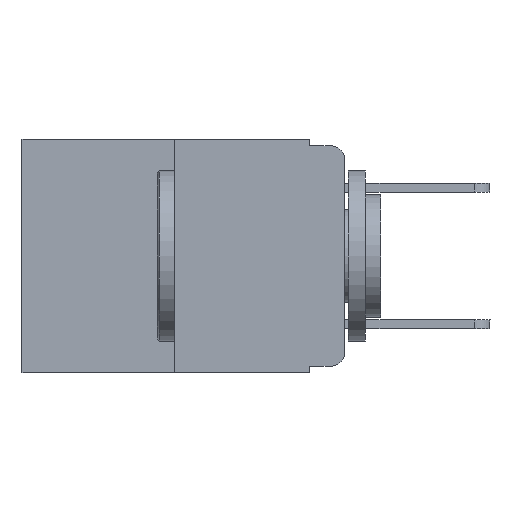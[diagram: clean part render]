
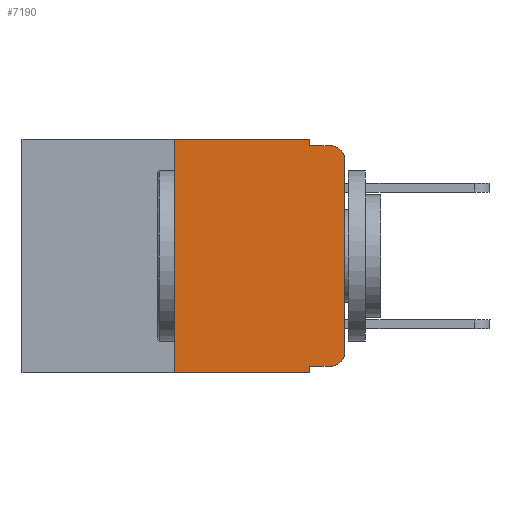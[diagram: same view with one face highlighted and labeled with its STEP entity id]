
A CAD part, left-side view. The second image highlights one B-rep face of the part: STEP entity #7190.
In plain terms, the highlighted planar face has unit normal (-1, 0, 0).
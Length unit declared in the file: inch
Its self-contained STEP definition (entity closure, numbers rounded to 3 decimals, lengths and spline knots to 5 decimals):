
#193 = CARTESIAN_POINT ( 'NONE',  ( 0., 0.02, -0.313 ) ) ;
#460 = VERTEX_POINT ( 'NONE', #11125 ) ;
#508 = VERTEX_POINT ( 'NONE', #9823 ) ;
#718 = DIRECTION ( 'NONE',  ( 0., -1., 0. ) ) ;
#870 = EDGE_CURVE ( 'NONE', #508, #15405, #17935, .T. ) ;
#947 = LINE ( 'NONE', #13880, #9600 ) ;
#1258 = EDGE_CURVE ( 'NONE', #11883, #17985, #17690, .T. ) ;
#1527 = LINE ( 'NONE', #17153, #15205 ) ;
#1578 = CARTESIAN_POINT ( 'NONE',  ( 0., 0.051, -0.01 ) ) ;
#1910 = ORIENTED_EDGE ( 'NONE', *, *, #1258, .T. ) ;
#2192 = VERTEX_POINT ( 'NONE', #6636 ) ;
#2486 = PLANE ( 'NONE',  #17309 ) ;
#2539 = CARTESIAN_POINT ( 'NONE',  ( 0., 0., -0.03 ) ) ;
#2745 = DIRECTION ( 'NONE',  ( 0., 0., -1. ) ) ;
#3162 = AXIS2_PLACEMENT_3D ( 'NONE', #193, #15656, #2745 ) ;
#3366 = ORIENTED_EDGE ( 'NONE', *, *, #870, .F. ) ;
#3822 = CARTESIAN_POINT ( 'NONE',  ( 0., 0.051, 0. ) ) ;
#4148 = ORIENTED_EDGE ( 'NONE', *, *, #4286, .F. ) ;
#4286 = EDGE_CURVE ( 'NONE', #15405, #4736, #947, .T. ) ;
#4331 = VECTOR ( 'NONE', #15826, 39.37008 ) ;
#4390 = EDGE_LOOP ( 'NONE', ( #16027, #1910, #17393, #4148, #3366, #5200, #5851, #8455, #18119, #8531 ) ) ;
#4405 = CARTESIAN_POINT ( 'NONE',  ( 0., 0., 0. ) ) ;
#4572 = CARTESIAN_POINT ( 'NONE',  ( 0., 0.051, -0.343 ) ) ;
#4736 = VERTEX_POINT ( 'NONE', #1578 ) ;
#4780 = EDGE_CURVE ( 'NONE', #4736, #17985, #13014, .T. ) ;
#4864 = DIRECTION ( 'NONE',  ( 0., -1., 0. ) ) ;
#4869 = AXIS2_PLACEMENT_3D ( 'NONE', #10899, #5118, #13799 ) ;
#5096 = VERTEX_POINT ( 'NONE', #18130 ) ;
#5118 = DIRECTION ( 'NONE',  ( -1., 0., 0. ) ) ;
#5120 = VECTOR ( 'NONE', #718, 39.37008 ) ;
#5200 = ORIENTED_EDGE ( 'NONE', *, *, #10684, .F. ) ;
#5493 = FACE_OUTER_BOUND ( 'NONE', #4390, .T. ) ;
#5517 = LINE ( 'NONE', #3822, #9323 ) ;
#5851 = ORIENTED_EDGE ( 'NONE', *, *, #15467, .T. ) ;
#5858 = DIRECTION ( 'NONE',  ( 0., -1., 0. ) ) ;
#6610 = CARTESIAN_POINT ( 'NONE',  ( 0., 0.473, 0. ) ) ;
#6636 = CARTESIAN_POINT ( 'NONE',  ( 0., 0.051, -0.333 ) ) ;
#6653 = EDGE_CURVE ( 'NONE', #2192, #18226, #5517, .T. ) ;
#6783 = CARTESIAN_POINT ( 'NONE',  ( 0., 0.051, 0. ) ) ;
#6886 = DIRECTION ( 'NONE',  ( 1., 0., 0. ) ) ;
#7190 = ADVANCED_FACE ( 'NONE', ( #5493 ), #2486, .F. ) ;
#7846 = CARTESIAN_POINT ( 'NONE',  ( 0., 0.473, 0. ) ) ;
#8426 = VECTOR ( 'NONE', #16928, 39.37008 ) ;
#8455 = ORIENTED_EDGE ( 'NONE', *, *, #6653, .F. ) ;
#8531 = ORIENTED_EDGE ( 'NONE', *, *, #10311, .T. ) ;
#8964 = LINE ( 'NONE', #16259, #17766 ) ;
#9323 = VECTOR ( 'NONE', #16731, 39.37008 ) ;
#9600 = VECTOR ( 'NONE', #12195, 39.37008 ) ;
#9823 = CARTESIAN_POINT ( 'NONE',  ( 0., 0.25, 0. ) ) ;
#10018 = CARTESIAN_POINT ( 'NONE',  ( 0., 0.25, 0. ) ) ;
#10093 = DIRECTION ( 'NONE',  ( 0., 0., 1. ) ) ;
#10311 = EDGE_CURVE ( 'NONE', #460, #5096, #12093, .T. ) ;
#10603 = VECTOR ( 'NONE', #10093, 39.37008 ) ;
#10684 = EDGE_CURVE ( 'NONE', #12792, #508, #12644, .T. ) ;
#10899 = CARTESIAN_POINT ( 'NONE',  ( 0., 0.02, -0.03 ) ) ;
#11125 = CARTESIAN_POINT ( 'NONE',  ( 0., 0.02, -0.333 ) ) ;
#11267 = EDGE_CURVE ( 'NONE', #5096, #11883, #12816, .T. ) ;
#11391 = EDGE_CURVE ( 'NONE', #2192, #460, #8964, .T. ) ;
#11883 = VERTEX_POINT ( 'NONE', #2539 ) ;
#12093 = CIRCLE ( 'NONE', #3162, 0.02 ) ;
#12195 = DIRECTION ( 'NONE',  ( 0., 0., -1. ) ) ;
#12415 = CARTESIAN_POINT ( 'NONE',  ( 0., 0.25, -0.343 ) ) ;
#12597 = DIRECTION ( 'NONE',  ( 0., 0., -1. ) ) ;
#12644 = LINE ( 'NONE', #10018, #4331 ) ;
#12792 = VERTEX_POINT ( 'NONE', #12415 ) ;
#12816 = LINE ( 'NONE', #4405, #10603 ) ;
#13014 = LINE ( 'NONE', #15444, #8426 ) ;
#13799 = DIRECTION ( 'NONE',  ( 0., 0., -1. ) ) ;
#13880 = CARTESIAN_POINT ( 'NONE',  ( 0., 0.051, 0. ) ) ;
#15205 = VECTOR ( 'NONE', #5858, 39.37008 ) ;
#15405 = VERTEX_POINT ( 'NONE', #6783 ) ;
#15444 = CARTESIAN_POINT ( 'NONE',  ( 0., 0.051, -0.01 ) ) ;
#15467 = EDGE_CURVE ( 'NONE', #12792, #18226, #1527, .T. ) ;
#15656 = DIRECTION ( 'NONE',  ( -1., 0., 0. ) ) ;
#15826 = DIRECTION ( 'NONE',  ( 0., 0., 1. ) ) ;
#16027 = ORIENTED_EDGE ( 'NONE', *, *, #11267, .T. ) ;
#16259 = CARTESIAN_POINT ( 'NONE',  ( 0., 0.051, -0.333 ) ) ;
#16731 = DIRECTION ( 'NONE',  ( 0., 0., -1. ) ) ;
#16928 = DIRECTION ( 'NONE',  ( 0., -1., 0. ) ) ;
#17153 = CARTESIAN_POINT ( 'NONE',  ( 0., 0.473, -0.343 ) ) ;
#17309 = AXIS2_PLACEMENT_3D ( 'NONE', #6610, #6886, #12597 ) ;
#17393 = ORIENTED_EDGE ( 'NONE', *, *, #4780, .F. ) ;
#17589 = CARTESIAN_POINT ( 'NONE',  ( 0., 0.02, -0.01 ) ) ;
#17690 = CIRCLE ( 'NONE', #4869, 0.02 ) ;
#17766 = VECTOR ( 'NONE', #4864, 39.37008 ) ;
#17935 = LINE ( 'NONE', #7846, #5120 ) ;
#17985 = VERTEX_POINT ( 'NONE', #17589 ) ;
#18119 = ORIENTED_EDGE ( 'NONE', *, *, #11391, .T. ) ;
#18130 = CARTESIAN_POINT ( 'NONE',  ( 0., 0., -0.313 ) ) ;
#18226 = VERTEX_POINT ( 'NONE', #4572 ) ;
